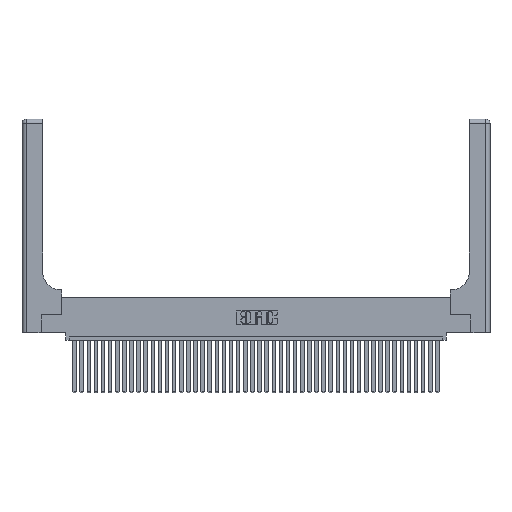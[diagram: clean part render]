
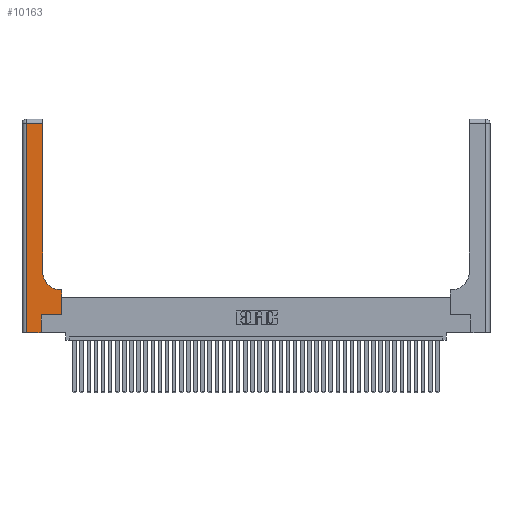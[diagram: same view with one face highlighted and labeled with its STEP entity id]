
A CAD part, top view. The second image highlights one B-rep face of the part: STEP entity #10163.
In plain terms, the highlighted planar face has unit normal (0, 0, 1).
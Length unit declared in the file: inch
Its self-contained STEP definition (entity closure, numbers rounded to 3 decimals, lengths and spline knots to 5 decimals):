
#130 = FACE_OUTER_BOUND ( 'NONE', #22907, .T. ) ;
#576 = DIRECTION ( 'NONE',  ( 0., 0., -1. ) ) ;
#1145 = CARTESIAN_POINT ( 'NONE',  ( 0.5585, 0.6, 0.37 ) ) ;
#1275 = EDGE_CURVE ( 'NONE', #23813, #16031, #4181, .T. ) ;
#1630 = VECTOR ( 'NONE', #33503, 39.37008 ) ;
#2324 = EDGE_CURVE ( 'NONE', #3011, #37371, #35871, .T. ) ;
#2570 = LINE ( 'NONE', #16779, #4633 ) ;
#2680 = AXIS2_PLACEMENT_3D ( 'NONE', #17245, #576, #7970 ) ;
#2960 = CARTESIAN_POINT ( 'NONE',  ( 0.2915, 0.6, 0.37 ) ) ;
#3011 = VERTEX_POINT ( 'NONE', #38873 ) ;
#4181 = CIRCLE ( 'NONE', #31597, 0.25 ) ;
#4633 = VECTOR ( 'NONE', #10251, 39.37008 ) ;
#5967 = CARTESIAN_POINT ( 'NONE',  ( 0.06, 0., 0.37 ) ) ;
#6191 = VERTEX_POINT ( 'NONE', #19502 ) ;
#7119 = VECTOR ( 'NONE', #39601, 39.37008 ) ;
#7970 = DIRECTION ( 'NONE',  ( -1., 0., 0. ) ) ;
#9496 = ORIENTED_EDGE ( 'NONE', *, *, #1275, .T. ) ;
#9574 = DIRECTION ( 'NONE',  ( 1., 0., 0. ) ) ;
#10163 = ADVANCED_FACE ( 'NONE', ( #130 ), #39988, .F. ) ;
#10251 = DIRECTION ( 'NONE',  ( -1., 0., 0. ) ) ;
#10640 = VERTEX_POINT ( 'NONE', #20097 ) ;
#10758 = CARTESIAN_POINT ( 'NONE',  ( 0., 0., 0.37 ) ) ;
#11013 = EDGE_CURVE ( 'NONE', #24322, #34231, #35459, .T. ) ;
#11855 = VECTOR ( 'NONE', #13624, 39.37008 ) ;
#12599 = CARTESIAN_POINT ( 'NONE',  ( 0.269, 0.25, 0.37 ) ) ;
#13624 = DIRECTION ( 'NONE',  ( 0., 1., 0. ) ) ;
#13696 = CARTESIAN_POINT ( 'NONE',  ( 0.269, 0., 0.37 ) ) ;
#14073 = DIRECTION ( 'NONE',  ( 1., 0., 0. ) ) ;
#14957 = EDGE_CURVE ( 'NONE', #10640, #3011, #38421, .T. ) ;
#16031 = VERTEX_POINT ( 'NONE', #35363 ) ;
#16779 = CARTESIAN_POINT ( 'NONE',  ( 0., 2.94, 0.37 ) ) ;
#16917 = EDGE_CURVE ( 'NONE', #37371, #23813, #33563, .T. ) ;
#16937 = ORIENTED_EDGE ( 'NONE', *, *, #16917, .T. ) ;
#17245 = CARTESIAN_POINT ( 'NONE',  ( 0., 3., 0.37 ) ) ;
#19502 = CARTESIAN_POINT ( 'NONE',  ( 0.06, 2.94, 0.37 ) ) ;
#19740 = CARTESIAN_POINT ( 'NONE',  ( 0.2915, 3., 0.37 ) ) ;
#20033 = EDGE_CURVE ( 'NONE', #40692, #6191, #2570, .T. ) ;
#20097 = CARTESIAN_POINT ( 'NONE',  ( 0.269, 0.25, 0.37 ) ) ;
#20685 = LINE ( 'NONE', #19740, #11855 ) ;
#21506 = CARTESIAN_POINT ( 'NONE',  ( 0.5585, 0.25, 0.37 ) ) ;
#22907 = EDGE_LOOP ( 'NONE', ( #33736, #28202, #27245, #41309, #31429, #32321, #29279, #16937, #9496 ) ) ;
#23800 = DIRECTION ( 'NONE',  ( 0., 1., 0. ) ) ;
#23813 = VERTEX_POINT ( 'NONE', #27697 ) ;
#24322 = VERTEX_POINT ( 'NONE', #5967 ) ;
#24692 = CARTESIAN_POINT ( 'NONE',  ( 0.2915, 2.94, 0.37 ) ) ;
#26832 = EDGE_CURVE ( 'NONE', #34231, #10640, #31714, .T. ) ;
#27245 = ORIENTED_EDGE ( 'NONE', *, *, #27330, .T. ) ;
#27330 = EDGE_CURVE ( 'NONE', #6191, #24322, #28071, .T. ) ;
#27697 = CARTESIAN_POINT ( 'NONE',  ( 0.5415, 0.6, 0.37 ) ) ;
#28071 = LINE ( 'NONE', #42771, #1630 ) ;
#28202 = ORIENTED_EDGE ( 'NONE', *, *, #20033, .T. ) ;
#29157 = VECTOR ( 'NONE', #23800, 39.37008 ) ;
#29279 = ORIENTED_EDGE ( 'NONE', *, *, #2324, .T. ) ;
#31429 = ORIENTED_EDGE ( 'NONE', *, *, #26832, .T. ) ;
#31597 = AXIS2_PLACEMENT_3D ( 'NONE', #31666, #38353, #35169 ) ;
#31666 = CARTESIAN_POINT ( 'NONE',  ( 0.5415, 0.85, 0.37 ) ) ;
#31714 = LINE ( 'NONE', #13696, #29157 ) ;
#32321 = ORIENTED_EDGE ( 'NONE', *, *, #14957, .T. ) ;
#33503 = DIRECTION ( 'NONE',  ( 0., -1., 0. ) ) ;
#33563 = LINE ( 'NONE', #2960, #7119 ) ;
#33736 = ORIENTED_EDGE ( 'NONE', *, *, #39826, .T. ) ;
#34231 = VERTEX_POINT ( 'NONE', #38437 ) ;
#34984 = DIRECTION ( 'NONE',  ( 0., 1., 0. ) ) ;
#35169 = DIRECTION ( 'NONE',  ( 1., 0., 0. ) ) ;
#35363 = CARTESIAN_POINT ( 'NONE',  ( 0.2915, 0.85, 0.37 ) ) ;
#35459 = LINE ( 'NONE', #10758, #41685 ) ;
#35871 = LINE ( 'NONE', #21506, #41026 ) ;
#36328 = VECTOR ( 'NONE', #9574, 39.37008 ) ;
#37371 = VERTEX_POINT ( 'NONE', #1145 ) ;
#38353 = DIRECTION ( 'NONE',  ( 0., 0., -1. ) ) ;
#38421 = LINE ( 'NONE', #12599, #36328 ) ;
#38437 = CARTESIAN_POINT ( 'NONE',  ( 0.269, 0., 0.37 ) ) ;
#38873 = CARTESIAN_POINT ( 'NONE',  ( 0.5585, 0.25, 0.37 ) ) ;
#39601 = DIRECTION ( 'NONE',  ( -1., 0., 0. ) ) ;
#39826 = EDGE_CURVE ( 'NONE', #16031, #40692, #20685, .T. ) ;
#39988 = PLANE ( 'NONE',  #2680 ) ;
#40692 = VERTEX_POINT ( 'NONE', #24692 ) ;
#41026 = VECTOR ( 'NONE', #34984, 39.37008 ) ;
#41309 = ORIENTED_EDGE ( 'NONE', *, *, #11013, .T. ) ;
#41685 = VECTOR ( 'NONE', #14073, 39.37008 ) ;
#42771 = CARTESIAN_POINT ( 'NONE',  ( 0.06, 3., 0.37 ) ) ;
